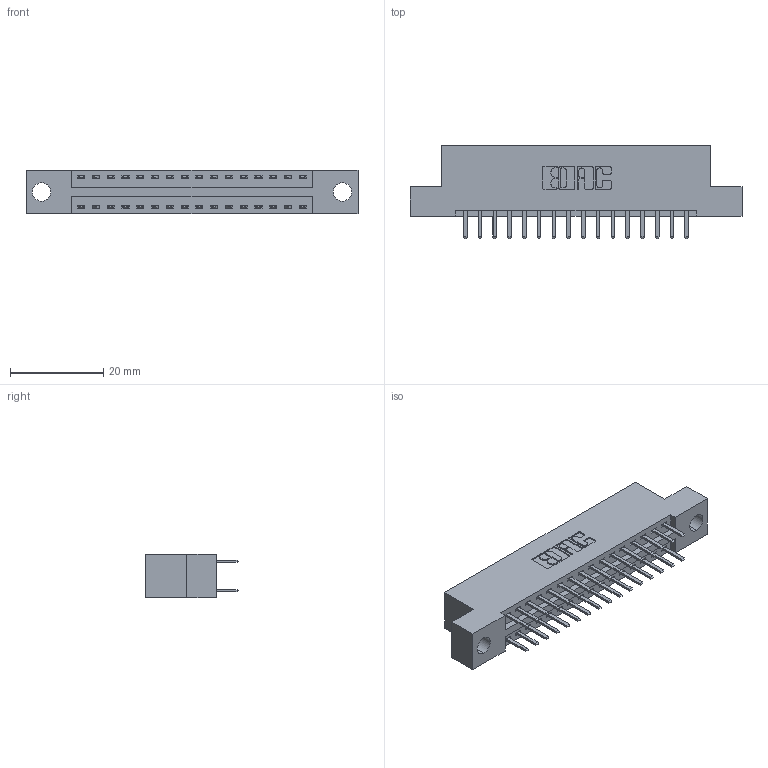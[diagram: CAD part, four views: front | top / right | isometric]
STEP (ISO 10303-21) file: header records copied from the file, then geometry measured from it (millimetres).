
FILE_DESCRIPTION (( 'STEP AP203' ), '1' );
FILE_NAME ('346-032-520-204.STEP', '2022-05-19T17:28:41', ( '' ), ( '' ), 'SwSTEP 2.0', 'SolidWorks 2020', '' );
FILE_SCHEMA (( 'CONFIG_CONTROL_DESIGN' ));
Length unit declared in the file: inch
Products named in the file (3): 345-292-001_345-293-120; 346-032-520-204; 346 Part_Flush Mounting Lugs - 0.156 Dia-TH
Assembly tree (33 placements, depth 2):
  346-032-520-204
    346 Part_Flush Mounting Lugs - 0.156 Dia-TH
    345-292-001_345-293-120  x32
Bounding box: 71.37 x 20.02 x 9.4 mm (x, y, z)
Volume: 6637.9 mm3; surface area: 8530.5 mm2
Topology: 33 solids, 33 shells, 1928 faces, 5581 edges, 3634 vertices
Faces by surface type: plane 1274, cylinder 654
Entity records: 14475 total; most frequent: CARTESIAN_POINT 2438, ORIENTED_EDGE 2358, DIRECTION 2187, EDGE_CURVE 1179, VECTOR 979, LINE 979, VERTEX_POINT 782, AXIS2_PLACEMENT_3D 604
